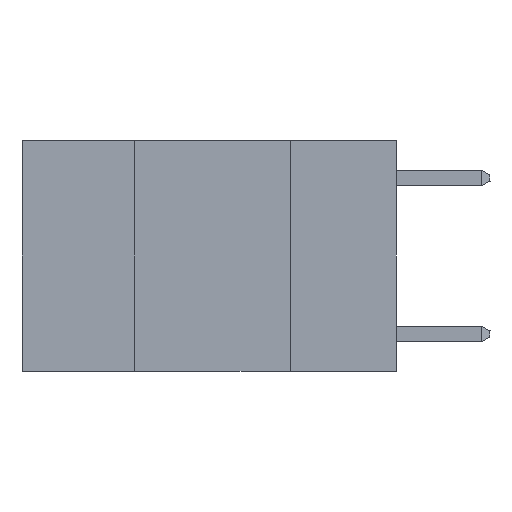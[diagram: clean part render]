
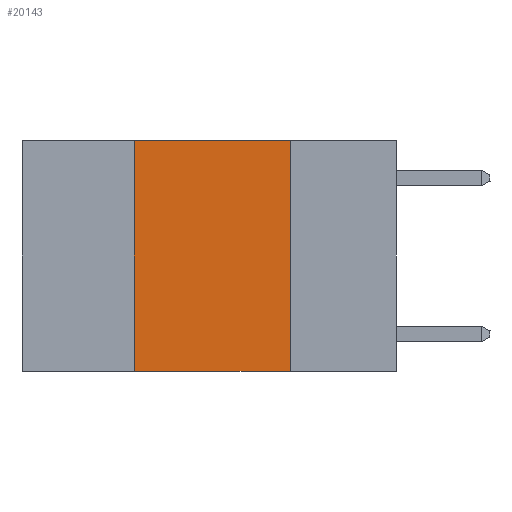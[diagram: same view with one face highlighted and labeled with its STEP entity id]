
A CAD part, left-side view. The second image highlights one B-rep face of the part: STEP entity #20143.
In plain terms, the highlighted planar face has unit normal (-1, 0, 0).
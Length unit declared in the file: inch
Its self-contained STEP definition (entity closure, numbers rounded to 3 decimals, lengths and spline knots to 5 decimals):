
#617 = CARTESIAN_POINT ( 'NONE',  ( 0., 0.6, 0. ) ) ;
#1130 = CARTESIAN_POINT ( 'NONE',  ( 0., 0.42, 0. ) ) ;
#1438 = DIRECTION ( 'NONE',  ( 0., -1., 0. ) ) ;
#1495 = VECTOR ( 'NONE', #20573, 39.37008 ) ;
#2335 = EDGE_CURVE ( 'NONE', #15743, #24057, #3775, .T. ) ;
#2632 = EDGE_CURVE ( 'NONE', #6063, #24057, #12087, .T. ) ;
#3775 = LINE ( 'NONE', #8121, #9466 ) ;
#4123 = CARTESIAN_POINT ( 'NONE',  ( 0., 0.17, -0.37 ) ) ;
#5494 = FACE_OUTER_BOUND ( 'NONE', #17873, .T. ) ;
#6063 = VERTEX_POINT ( 'NONE', #19780 ) ;
#6387 = CARTESIAN_POINT ( 'NONE',  ( 0., 0.42, -0.37 ) ) ;
#7019 = DIRECTION ( 'NONE',  ( 0., 0., -1. ) ) ;
#8121 = CARTESIAN_POINT ( 'NONE',  ( 0., 0.6, -0.37 ) ) ;
#8133 = AXIS2_PLACEMENT_3D ( 'NONE', #617, #19627, #7019 ) ;
#8400 = VERTEX_POINT ( 'NONE', #1130 ) ;
#9466 = VECTOR ( 'NONE', #21174, 39.37008 ) ;
#9869 = VECTOR ( 'NONE', #1438, 39.37008 ) ;
#9903 = EDGE_CURVE ( 'NONE', #8400, #6063, #10519, .T. ) ;
#10519 = LINE ( 'NONE', #24408, #9869 ) ;
#11118 = LINE ( 'NONE', #24025, #21773 ) ;
#12087 = LINE ( 'NONE', #21077, #1495 ) ;
#13288 = ORIENTED_EDGE ( 'NONE', *, *, #2632, .F. ) ;
#13676 = DIRECTION ( 'NONE',  ( 0., 0., 1. ) ) ;
#14072 = ORIENTED_EDGE ( 'NONE', *, *, #9903, .F. ) ;
#15743 = VERTEX_POINT ( 'NONE', #6387 ) ;
#16029 = EDGE_CURVE ( 'NONE', #15743, #8400, #11118, .T. ) ;
#17021 = ORIENTED_EDGE ( 'NONE', *, *, #16029, .F. ) ;
#17541 = PLANE ( 'NONE',  #8133 ) ;
#17873 = EDGE_LOOP ( 'NONE', ( #13288, #14072, #17021, #18875 ) ) ;
#18875 = ORIENTED_EDGE ( 'NONE', *, *, #2335, .T. ) ;
#19627 = DIRECTION ( 'NONE',  ( 1., 0., 0. ) ) ;
#19780 = CARTESIAN_POINT ( 'NONE',  ( 0., 0.17, 0. ) ) ;
#20143 = ADVANCED_FACE ( 'NONE', ( #5494 ), #17541, .F. ) ;
#20573 = DIRECTION ( 'NONE',  ( 0., 0., -1. ) ) ;
#21077 = CARTESIAN_POINT ( 'NONE',  ( 0., 0.17, 0. ) ) ;
#21174 = DIRECTION ( 'NONE',  ( 0., -1., 0. ) ) ;
#21773 = VECTOR ( 'NONE', #13676, 39.37008 ) ;
#24025 = CARTESIAN_POINT ( 'NONE',  ( 0., 0.42, 0. ) ) ;
#24057 = VERTEX_POINT ( 'NONE', #4123 ) ;
#24408 = CARTESIAN_POINT ( 'NONE',  ( 0., 0.6, 0. ) ) ;
